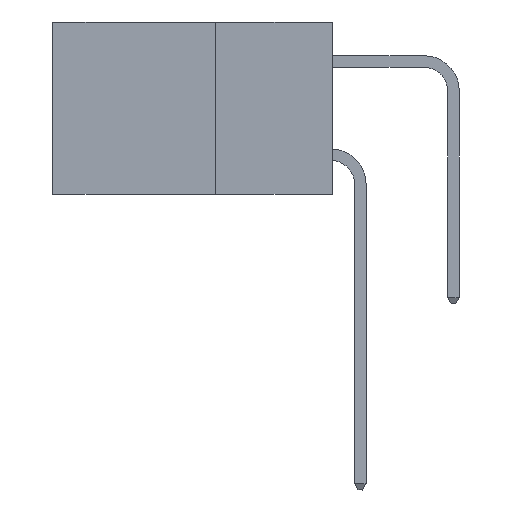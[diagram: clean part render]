
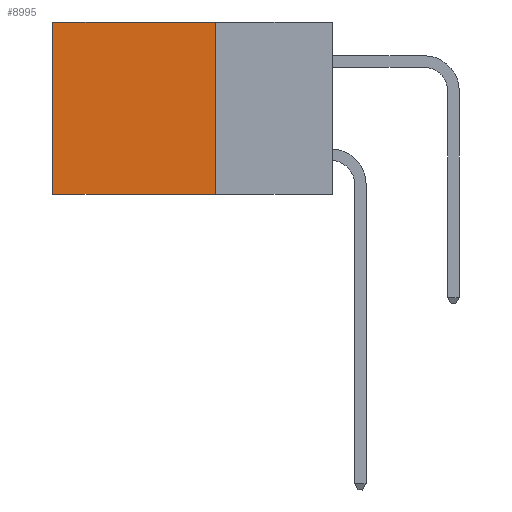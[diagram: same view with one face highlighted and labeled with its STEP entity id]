
A CAD part, left-side view. The second image highlights one B-rep face of the part: STEP entity #8995.
In plain terms, the highlighted planar face has unit normal (-1, 0, 0).
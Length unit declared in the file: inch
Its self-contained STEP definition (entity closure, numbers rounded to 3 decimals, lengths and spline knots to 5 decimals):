
#1296 = EDGE_LOOP ( 'NONE', ( #12168, #3141, #4014, #6124 ) ) ;
#1750 = VERTEX_POINT ( 'NONE', #3148 ) ;
#1939 = FACE_OUTER_BOUND ( 'NONE', #1296, .T. ) ;
#2649 = LINE ( 'NONE', #7097, #14637 ) ;
#2707 = LINE ( 'NONE', #3310, #18560 ) ;
#3141 = ORIENTED_EDGE ( 'NONE', *, *, #4915, .F. ) ;
#3148 = CARTESIAN_POINT ( 'NONE',  ( 0.298, 0.25, -0.37 ) ) ;
#3310 = CARTESIAN_POINT ( 'NONE',  ( 0.298, 0.25, 0. ) ) ;
#4014 = ORIENTED_EDGE ( 'NONE', *, *, #5555, .F. ) ;
#4371 = AXIS2_PLACEMENT_3D ( 'NONE', #8582, #18964, #10078 ) ;
#4915 = EDGE_CURVE ( 'NONE', #1750, #14104, #10900, .T. ) ;
#4988 = VERTEX_POINT ( 'NONE', #7121 ) ;
#5115 = LINE ( 'NONE', #7530, #8611 ) ;
#5451 = CARTESIAN_POINT ( 'NONE',  ( 0.298, 0.6, -0.37 ) ) ;
#5555 = EDGE_CURVE ( 'NONE', #4988, #1750, #2649, .T. ) ;
#6124 = ORIENTED_EDGE ( 'NONE', *, *, #17383, .T. ) ;
#6434 = VECTOR ( 'NONE', #11385, 39.37008 ) ;
#7097 = CARTESIAN_POINT ( 'NONE',  ( 0.298, 0.25, 0. ) ) ;
#7121 = CARTESIAN_POINT ( 'NONE',  ( 0.298, 0.25, 0. ) ) ;
#7530 = CARTESIAN_POINT ( 'NONE',  ( 0.298, 0.6, 0. ) ) ;
#8367 = CARTESIAN_POINT ( 'NONE',  ( 0.298, 0.6, 0. ) ) ;
#8582 = CARTESIAN_POINT ( 'NONE',  ( 0.298, 0.25, 0. ) ) ;
#8611 = VECTOR ( 'NONE', #9065, 39.37008 ) ;
#8995 = ADVANCED_FACE ( 'NONE', ( #1939 ), #16043, .F. ) ;
#9065 = DIRECTION ( 'NONE',  ( 0., 0., -1. ) ) ;
#10078 = DIRECTION ( 'NONE',  ( 0., 0., -1. ) ) ;
#10900 = LINE ( 'NONE', #17363, #6434 ) ;
#11385 = DIRECTION ( 'NONE',  ( 0., 1., 0. ) ) ;
#12168 = ORIENTED_EDGE ( 'NONE', *, *, #15388, .T. ) ;
#12737 = VERTEX_POINT ( 'NONE', #8367 ) ;
#13781 = DIRECTION ( 'NONE',  ( 0., 1., 0. ) ) ;
#14104 = VERTEX_POINT ( 'NONE', #5451 ) ;
#14637 = VECTOR ( 'NONE', #17532, 39.37008 ) ;
#15388 = EDGE_CURVE ( 'NONE', #12737, #14104, #5115, .T. ) ;
#16043 = PLANE ( 'NONE',  #4371 ) ;
#17363 = CARTESIAN_POINT ( 'NONE',  ( 0.298, 0.25, -0.37 ) ) ;
#17383 = EDGE_CURVE ( 'NONE', #4988, #12737, #2707, .T. ) ;
#17532 = DIRECTION ( 'NONE',  ( 0., 0., -1. ) ) ;
#18560 = VECTOR ( 'NONE', #13781, 39.37008 ) ;
#18964 = DIRECTION ( 'NONE',  ( 1., 0., 0. ) ) ;
